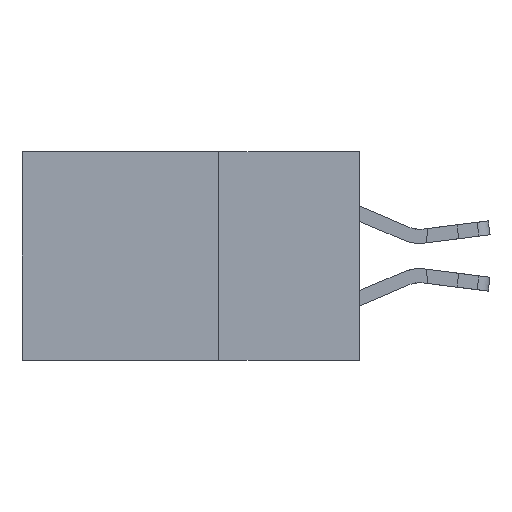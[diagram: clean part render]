
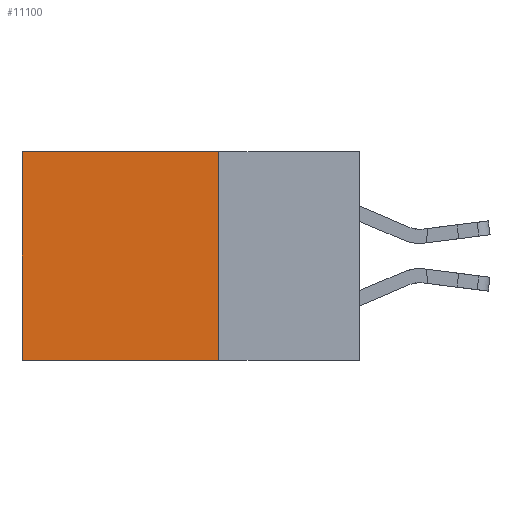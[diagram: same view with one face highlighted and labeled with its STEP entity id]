
A CAD part, left-side view. The second image highlights one B-rep face of the part: STEP entity #11100.
In plain terms, the highlighted planar face has unit normal (-1, 0, 0).
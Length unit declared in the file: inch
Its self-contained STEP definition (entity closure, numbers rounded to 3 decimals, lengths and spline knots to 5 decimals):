
#2019 = CARTESIAN_POINT ( 'NONE',  ( 0.2875, 0.25, -0.37 ) ) ;
#2444 = EDGE_CURVE ( 'NONE', #25051, #7652, #12015, .T. ) ;
#2757 = EDGE_CURVE ( 'NONE', #21989, #25051, #12629, .T. ) ;
#2893 = DIRECTION ( 'NONE',  ( 0., 0., -1. ) ) ;
#3610 = CARTESIAN_POINT ( 'NONE',  ( 0.2875, 0.6, 0. ) ) ;
#5883 = CARTESIAN_POINT ( 'NONE',  ( 0.2875, 0.25, -0.37 ) ) ;
#7166 = EDGE_LOOP ( 'NONE', ( #11244, #22824, #23248, #17092 ) ) ;
#7282 = VECTOR ( 'NONE', #23509, 39.37008 ) ;
#7652 = VERTEX_POINT ( 'NONE', #21914 ) ;
#7791 = AXIS2_PLACEMENT_3D ( 'NONE', #20185, #18265, #16598 ) ;
#9035 = VERTEX_POINT ( 'NONE', #24715 ) ;
#10443 = EDGE_CURVE ( 'NONE', #21989, #9035, #11079, .T. ) ;
#11079 = LINE ( 'NONE', #12992, #22022 ) ;
#11100 = ADVANCED_FACE ( 'NONE', ( #23892 ), #18148, .F. ) ;
#11244 = ORIENTED_EDGE ( 'NONE', *, *, #20672, .T. ) ;
#11919 = CARTESIAN_POINT ( 'NONE',  ( 0.2875, 0.25, 0. ) ) ;
#12015 = LINE ( 'NONE', #5883, #7282 ) ;
#12629 = LINE ( 'NONE', #20409, #23437 ) ;
#12992 = CARTESIAN_POINT ( 'NONE',  ( 0.2875, 0.25, 0. ) ) ;
#13224 = DIRECTION ( 'NONE',  ( 0., 0., -1. ) ) ;
#16598 = DIRECTION ( 'NONE',  ( 0., 0., -1. ) ) ;
#17092 = ORIENTED_EDGE ( 'NONE', *, *, #10443, .T. ) ;
#18148 = PLANE ( 'NONE',  #7791 ) ;
#18265 = DIRECTION ( 'NONE',  ( 1., 0., 0. ) ) ;
#20185 = CARTESIAN_POINT ( 'NONE',  ( 0.2875, 0.25, 0. ) ) ;
#20409 = CARTESIAN_POINT ( 'NONE',  ( 0.2875, 0.25, 0. ) ) ;
#20525 = DIRECTION ( 'NONE',  ( 0., 1., 0. ) ) ;
#20672 = EDGE_CURVE ( 'NONE', #9035, #7652, #21125, .T. ) ;
#21125 = LINE ( 'NONE', #3610, #22854 ) ;
#21914 = CARTESIAN_POINT ( 'NONE',  ( 0.2875, 0.6, -0.37 ) ) ;
#21989 = VERTEX_POINT ( 'NONE', #11919 ) ;
#22022 = VECTOR ( 'NONE', #20525, 39.37008 ) ;
#22824 = ORIENTED_EDGE ( 'NONE', *, *, #2444, .F. ) ;
#22854 = VECTOR ( 'NONE', #13224, 39.37008 ) ;
#23248 = ORIENTED_EDGE ( 'NONE', *, *, #2757, .F. ) ;
#23437 = VECTOR ( 'NONE', #2893, 39.37008 ) ;
#23509 = DIRECTION ( 'NONE',  ( 0., 1., 0. ) ) ;
#23892 = FACE_OUTER_BOUND ( 'NONE', #7166, .T. ) ;
#24715 = CARTESIAN_POINT ( 'NONE',  ( 0.2875, 0.6, 0. ) ) ;
#25051 = VERTEX_POINT ( 'NONE', #2019 ) ;
